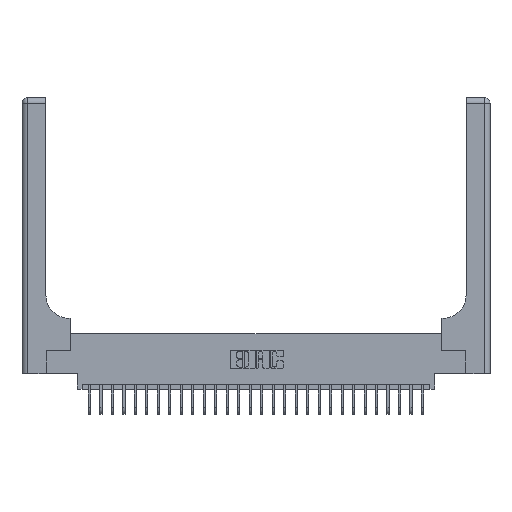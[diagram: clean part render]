
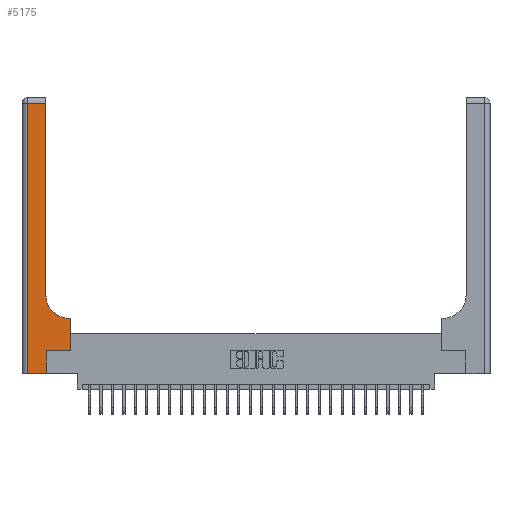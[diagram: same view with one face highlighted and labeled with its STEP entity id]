
A CAD part, top view. The second image highlights one B-rep face of the part: STEP entity #5175.
In plain terms, the highlighted planar face has unit normal (0, 0, 1).
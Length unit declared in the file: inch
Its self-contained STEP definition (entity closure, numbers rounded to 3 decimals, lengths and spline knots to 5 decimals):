
#105 = DIRECTION ( 'NONE',  ( 0., 0., -1. ) ) ;
#274 = EDGE_CURVE ( 'NONE', #22451, #8262, #27366, .T. ) ;
#687 = DIRECTION ( 'NONE',  ( 1., 0., 0. ) ) ;
#1236 = VERTEX_POINT ( 'NONE', #24519 ) ;
#1278 = CARTESIAN_POINT ( 'NONE',  ( 0.26, 0.6, 0.37 ) ) ;
#1846 = CIRCLE ( 'NONE', #5558, 0.25 ) ;
#2239 = EDGE_CURVE ( 'NONE', #1236, #5862, #4443, .T. ) ;
#2893 = ORIENTED_EDGE ( 'NONE', *, *, #9116, .T. ) ;
#3135 = LINE ( 'NONE', #20846, #6664 ) ;
#3898 = VECTOR ( 'NONE', #687, 39.37008 ) ;
#4182 = ORIENTED_EDGE ( 'NONE', *, *, #6249, .T. ) ;
#4220 = VECTOR ( 'NONE', #12883, 39.37008 ) ;
#4443 = LINE ( 'NONE', #17369, #4220 ) ;
#4688 = ORIENTED_EDGE ( 'NONE', *, *, #16509, .T. ) ;
#4900 = CARTESIAN_POINT ( 'NONE',  ( 0., 0., 0.37 ) ) ;
#5175 = ADVANCED_FACE ( 'NONE', ( #18434 ), #16395, .F. ) ;
#5558 = AXIS2_PLACEMENT_3D ( 'NONE', #13198, #105, #15091 ) ;
#5618 = EDGE_CURVE ( 'NONE', #20481, #22451, #3135, .T. ) ;
#5688 = AXIS2_PLACEMENT_3D ( 'NONE', #9998, #7374, #25102 ) ;
#5862 = VERTEX_POINT ( 'NONE', #24514 ) ;
#6249 = EDGE_CURVE ( 'NONE', #23699, #20481, #15349, .T. ) ;
#6264 = EDGE_LOOP ( 'NONE', ( #4182, #28216, #21550, #22181, #15680, #2893, #10975, #17274, #4688 ) ) ;
#6465 = VECTOR ( 'NONE', #21600, 39.37008 ) ;
#6664 = VECTOR ( 'NONE', #24931, 39.37008 ) ;
#6948 = DIRECTION ( 'NONE',  ( 0., 1., 0. ) ) ;
#7374 = DIRECTION ( 'NONE',  ( 0., 0., -1. ) ) ;
#7946 = LINE ( 'NONE', #8229, #6465 ) ;
#8229 = CARTESIAN_POINT ( 'NONE',  ( 0.265, 0.25, 0.37 ) ) ;
#8262 = VERTEX_POINT ( 'NONE', #18500 ) ;
#9116 = EDGE_CURVE ( 'NONE', #5862, #16796, #7946, .T. ) ;
#9998 = CARTESIAN_POINT ( 'NONE',  ( 0., 3., 0.37 ) ) ;
#10975 = ORIENTED_EDGE ( 'NONE', *, *, #21331, .T. ) ;
#12316 = LINE ( 'NONE', #1278, #19660 ) ;
#12883 = DIRECTION ( 'NONE',  ( 0., 1., 0. ) ) ;
#13198 = CARTESIAN_POINT ( 'NONE',  ( 0.51, 0.85, 0.37 ) ) ;
#13680 = VERTEX_POINT ( 'NONE', #19268 ) ;
#13727 = CARTESIAN_POINT ( 'NONE',  ( 0.06, 3., 0.37 ) ) ;
#14303 = VERTEX_POINT ( 'NONE', #26626 ) ;
#15091 = DIRECTION ( 'NONE',  ( 1., 0., 0. ) ) ;
#15349 = LINE ( 'NONE', #24203, #16919 ) ;
#15680 = ORIENTED_EDGE ( 'NONE', *, *, #2239, .T. ) ;
#16097 = LINE ( 'NONE', #4900, #3898 ) ;
#16395 = PLANE ( 'NONE',  #5688 ) ;
#16509 = EDGE_CURVE ( 'NONE', #13680, #23699, #1846, .T. ) ;
#16796 = VERTEX_POINT ( 'NONE', #23335 ) ;
#16919 = VECTOR ( 'NONE', #26528, 39.37008 ) ;
#17274 = ORIENTED_EDGE ( 'NONE', *, *, #21497, .T. ) ;
#17369 = CARTESIAN_POINT ( 'NONE',  ( 0.265, 0., 0.37 ) ) ;
#18005 = LINE ( 'NONE', #26874, #19200 ) ;
#18434 = FACE_OUTER_BOUND ( 'NONE', #6264, .T. ) ;
#18500 = CARTESIAN_POINT ( 'NONE',  ( 0.06, 0., 0.37 ) ) ;
#19200 = VECTOR ( 'NONE', #6948, 39.37008 ) ;
#19268 = CARTESIAN_POINT ( 'NONE',  ( 0.51, 0.6, 0.37 ) ) ;
#19333 = VECTOR ( 'NONE', #23121, 39.37008 ) ;
#19660 = VECTOR ( 'NONE', #27874, 39.37008 ) ;
#20481 = VERTEX_POINT ( 'NONE', #20542 ) ;
#20542 = CARTESIAN_POINT ( 'NONE',  ( 0.26, 2.94, 0.37 ) ) ;
#20846 = CARTESIAN_POINT ( 'NONE',  ( 0., 2.94, 0.37 ) ) ;
#21331 = EDGE_CURVE ( 'NONE', #16796, #14303, #18005, .T. ) ;
#21497 = EDGE_CURVE ( 'NONE', #14303, #13680, #12316, .T. ) ;
#21550 = ORIENTED_EDGE ( 'NONE', *, *, #274, .T. ) ;
#21600 = DIRECTION ( 'NONE',  ( 1., 0., 0. ) ) ;
#22181 = ORIENTED_EDGE ( 'NONE', *, *, #23172, .T. ) ;
#22451 = VERTEX_POINT ( 'NONE', #25613 ) ;
#23121 = DIRECTION ( 'NONE',  ( 0., -1., 0. ) ) ;
#23172 = EDGE_CURVE ( 'NONE', #8262, #1236, #16097, .T. ) ;
#23335 = CARTESIAN_POINT ( 'NONE',  ( 0.528, 0.25, 0.37 ) ) ;
#23699 = VERTEX_POINT ( 'NONE', #26816 ) ;
#24203 = CARTESIAN_POINT ( 'NONE',  ( 0.26, 3., 0.37 ) ) ;
#24514 = CARTESIAN_POINT ( 'NONE',  ( 0.265, 0.25, 0.37 ) ) ;
#24519 = CARTESIAN_POINT ( 'NONE',  ( 0.265, 0., 0.37 ) ) ;
#24931 = DIRECTION ( 'NONE',  ( -1., 0., 0. ) ) ;
#25102 = DIRECTION ( 'NONE',  ( -1., 0., 0. ) ) ;
#25613 = CARTESIAN_POINT ( 'NONE',  ( 0.06, 2.94, 0.37 ) ) ;
#26528 = DIRECTION ( 'NONE',  ( 0., 1., 0. ) ) ;
#26626 = CARTESIAN_POINT ( 'NONE',  ( 0.528, 0.6, 0.37 ) ) ;
#26816 = CARTESIAN_POINT ( 'NONE',  ( 0.26, 0.85, 0.37 ) ) ;
#26874 = CARTESIAN_POINT ( 'NONE',  ( 0.528, 0.25, 0.37 ) ) ;
#27366 = LINE ( 'NONE', #13727, #19333 ) ;
#27874 = DIRECTION ( 'NONE',  ( -1., 0., 0. ) ) ;
#28216 = ORIENTED_EDGE ( 'NONE', *, *, #5618, .T. ) ;
